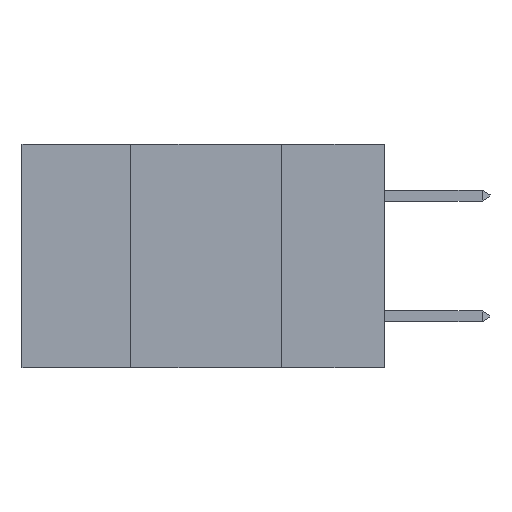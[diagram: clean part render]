
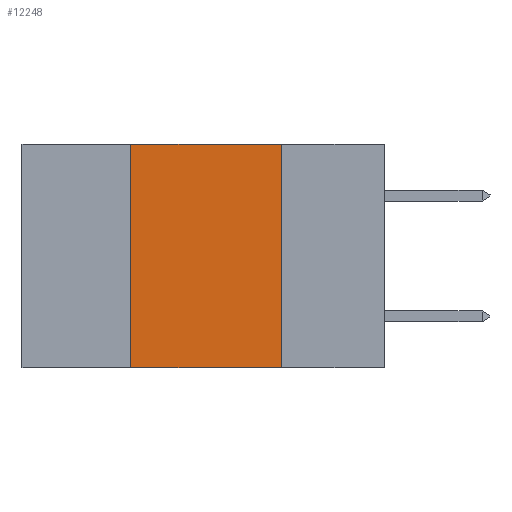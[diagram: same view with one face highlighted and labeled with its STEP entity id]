
A CAD part, left-side view. The second image highlights one B-rep face of the part: STEP entity #12248.
In plain terms, the highlighted planar face has unit normal (-1, 0, 0).
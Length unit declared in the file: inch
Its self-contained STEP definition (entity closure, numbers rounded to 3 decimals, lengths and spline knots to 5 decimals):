
#234 = VECTOR ( 'NONE', #13180, 39.37008 ) ;
#1006 = CARTESIAN_POINT ( 'NONE',  ( 0., 0.6, -0.37 ) ) ;
#1182 = LINE ( 'NONE', #1006, #10336 ) ;
#1212 = ORIENTED_EDGE ( 'NONE', *, *, #12483, .T. ) ;
#1426 = CARTESIAN_POINT ( 'NONE',  ( 0., 0.17, 0. ) ) ;
#2548 = EDGE_LOOP ( 'NONE', ( #4294, #17312, #13524, #1212 ) ) ;
#2704 = DIRECTION ( 'NONE',  ( 0., -1., 0. ) ) ;
#2900 = EDGE_CURVE ( 'NONE', #5249, #15567, #8020, .T. ) ;
#3202 = VECTOR ( 'NONE', #13602, 39.37008 ) ;
#4294 = ORIENTED_EDGE ( 'NONE', *, *, #2900, .F. ) ;
#4319 = PLANE ( 'NONE',  #6243 ) ;
#4579 = VECTOR ( 'NONE', #2704, 39.37008 ) ;
#5102 = CARTESIAN_POINT ( 'NONE',  ( 0., 0.17, 0. ) ) ;
#5249 = VERTEX_POINT ( 'NONE', #1426 ) ;
#6243 = AXIS2_PLACEMENT_3D ( 'NONE', #7138, #12719, #17940 ) ;
#6863 = FACE_OUTER_BOUND ( 'NONE', #2548, .T. ) ;
#7138 = CARTESIAN_POINT ( 'NONE',  ( 0., 0.6, 0. ) ) ;
#8020 = LINE ( 'NONE', #5102, #3202 ) ;
#8208 = DIRECTION ( 'NONE',  ( 0., -1., 0. ) ) ;
#10080 = VERTEX_POINT ( 'NONE', #16294 ) ;
#10336 = VECTOR ( 'NONE', #8208, 39.37008 ) ;
#10429 = LINE ( 'NONE', #14365, #234 ) ;
#12248 = ADVANCED_FACE ( 'NONE', ( #6863 ), #4319, .F. ) ;
#12483 = EDGE_CURVE ( 'NONE', #14625, #15567, #1182, .T. ) ;
#12719 = DIRECTION ( 'NONE',  ( 1., 0., 0. ) ) ;
#13180 = DIRECTION ( 'NONE',  ( 0., 0., 1. ) ) ;
#13524 = ORIENTED_EDGE ( 'NONE', *, *, #16126, .F. ) ;
#13602 = DIRECTION ( 'NONE',  ( 0., 0., -1. ) ) ;
#14365 = CARTESIAN_POINT ( 'NONE',  ( 0., 0.42, 0. ) ) ;
#14625 = VERTEX_POINT ( 'NONE', #16377 ) ;
#15195 = CARTESIAN_POINT ( 'NONE',  ( 0., 0.6, 0. ) ) ;
#15567 = VERTEX_POINT ( 'NONE', #15574 ) ;
#15574 = CARTESIAN_POINT ( 'NONE',  ( 0., 0.17, -0.37 ) ) ;
#15761 = EDGE_CURVE ( 'NONE', #10080, #5249, #17945, .T. ) ;
#16126 = EDGE_CURVE ( 'NONE', #14625, #10080, #10429, .T. ) ;
#16294 = CARTESIAN_POINT ( 'NONE',  ( 0., 0.42, 0. ) ) ;
#16377 = CARTESIAN_POINT ( 'NONE',  ( 0., 0.42, -0.37 ) ) ;
#17312 = ORIENTED_EDGE ( 'NONE', *, *, #15761, .F. ) ;
#17940 = DIRECTION ( 'NONE',  ( 0., 0., -1. ) ) ;
#17945 = LINE ( 'NONE', #15195, #4579 ) ;
